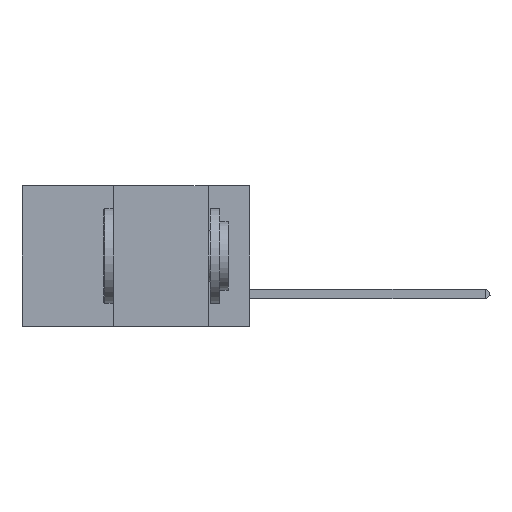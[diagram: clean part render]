
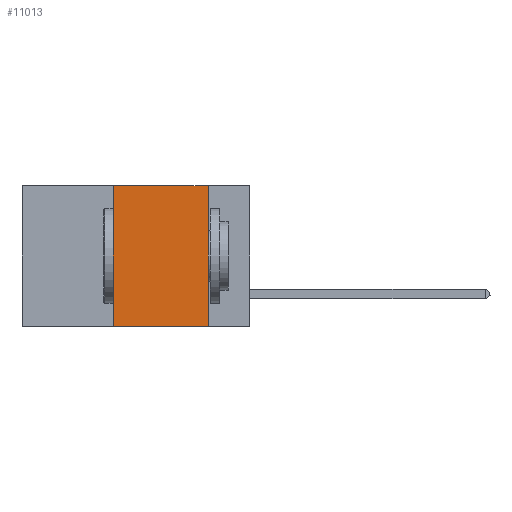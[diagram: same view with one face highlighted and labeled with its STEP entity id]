
A CAD part, left-side view. The second image highlights one B-rep face of the part: STEP entity #11013.
In plain terms, the highlighted planar face has unit normal (-1, 0, 0).
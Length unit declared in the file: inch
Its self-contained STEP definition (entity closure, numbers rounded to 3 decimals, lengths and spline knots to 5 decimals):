
#1448 = ORIENTED_EDGE ( 'NONE', *, *, #6773, .T. ) ;
#1514 = DIRECTION ( 'NONE',  ( 0., -1., 0. ) ) ;
#1752 = DIRECTION ( 'NONE',  ( 0., 0., -1. ) ) ;
#2001 = LINE ( 'NONE', #28028, #15815 ) ;
#2086 = LINE ( 'NONE', #28276, #6579 ) ;
#2872 = VERTEX_POINT ( 'NONE', #9853 ) ;
#2883 = LINE ( 'NONE', #13508, #15677 ) ;
#3385 = VECTOR ( 'NONE', #27447, 39.37008 ) ;
#5220 = DIRECTION ( 'NONE',  ( 1., 0., 0. ) ) ;
#6579 = VECTOR ( 'NONE', #1752, 39.37008 ) ;
#6773 = EDGE_CURVE ( 'NONE', #12961, #18229, #2001, .T. ) ;
#7353 = PLANE ( 'NONE',  #23238 ) ;
#8217 = LINE ( 'NONE', #11345, #3385 ) ;
#9555 = ORIENTED_EDGE ( 'NONE', *, *, #26348, .F. ) ;
#9853 = CARTESIAN_POINT ( 'NONE',  ( 0., 0.11, 0. ) ) ;
#11013 = ADVANCED_FACE ( 'NONE', ( #12205 ), #7353, .F. ) ;
#11345 = CARTESIAN_POINT ( 'NONE',  ( 0., 0.36, 0. ) ) ;
#12205 = FACE_OUTER_BOUND ( 'NONE', #21012, .T. ) ;
#12961 = VERTEX_POINT ( 'NONE', #27665 ) ;
#13426 = DIRECTION ( 'NONE',  ( 0., -1., 0. ) ) ;
#13508 = CARTESIAN_POINT ( 'NONE',  ( 0., 0.6, 0. ) ) ;
#15347 = ORIENTED_EDGE ( 'NONE', *, *, #22585, .F. ) ;
#15677 = VECTOR ( 'NONE', #13426, 39.37008 ) ;
#15815 = VECTOR ( 'NONE', #1514, 39.37008 ) ;
#16447 = VERTEX_POINT ( 'NONE', #16709 ) ;
#16709 = CARTESIAN_POINT ( 'NONE',  ( 0., 0.36, 0. ) ) ;
#17999 = ORIENTED_EDGE ( 'NONE', *, *, #27422, .F. ) ;
#18229 = VERTEX_POINT ( 'NONE', #23902 ) ;
#20433 = DIRECTION ( 'NONE',  ( 0., 0., -1. ) ) ;
#21012 = EDGE_LOOP ( 'NONE', ( #17999, #15347, #9555, #1448 ) ) ;
#22585 = EDGE_CURVE ( 'NONE', #16447, #2872, #2883, .T. ) ;
#23238 = AXIS2_PLACEMENT_3D ( 'NONE', #27025, #5220, #20433 ) ;
#23902 = CARTESIAN_POINT ( 'NONE',  ( 0., 0.11, -0.37 ) ) ;
#26348 = EDGE_CURVE ( 'NONE', #12961, #16447, #8217, .T. ) ;
#27025 = CARTESIAN_POINT ( 'NONE',  ( 0., 0.6, 0. ) ) ;
#27422 = EDGE_CURVE ( 'NONE', #2872, #18229, #2086, .T. ) ;
#27447 = DIRECTION ( 'NONE',  ( 0., 0., 1. ) ) ;
#27665 = CARTESIAN_POINT ( 'NONE',  ( 0., 0.36, -0.37 ) ) ;
#28028 = CARTESIAN_POINT ( 'NONE',  ( 0., 0.6, -0.37 ) ) ;
#28276 = CARTESIAN_POINT ( 'NONE',  ( 0., 0.11, 0. ) ) ;
